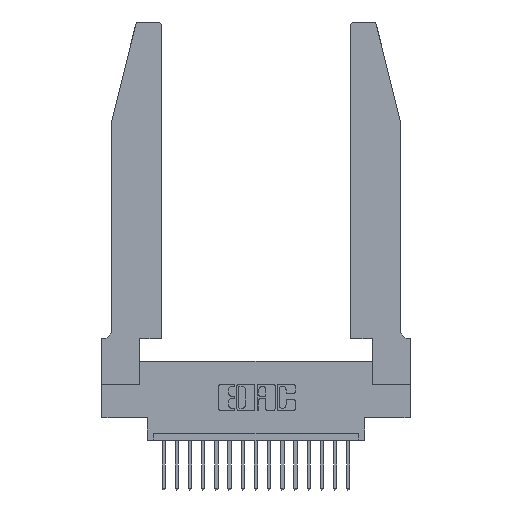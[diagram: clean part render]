
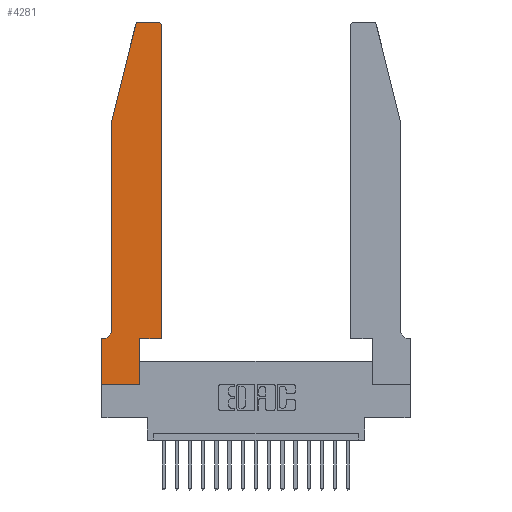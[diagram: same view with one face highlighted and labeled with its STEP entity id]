
A CAD part, top view. The second image highlights one B-rep face of the part: STEP entity #4281.
In plain terms, the highlighted planar face has unit normal (0, 0, 1).
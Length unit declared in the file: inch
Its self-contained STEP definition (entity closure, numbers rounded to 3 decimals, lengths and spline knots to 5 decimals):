
#148 = DIRECTION ( 'NONE',  ( 1., 0., 0. ) ) ;
#399 = CARTESIAN_POINT ( 'NONE',  ( 0., 0., 0.37 ) ) ;
#440 = ORIENTED_EDGE ( 'NONE', *, *, #5815, .T. ) ;
#626 = CARTESIAN_POINT ( 'NONE',  ( 0.4205, 2.75, 0.37 ) ) ;
#705 = CARTESIAN_POINT ( 'NONE',  ( 0.2865, 0., 0.37 ) ) ;
#860 = FACE_OUTER_BOUND ( 'NONE', #7319, .T. ) ;
#885 = VECTOR ( 'NONE', #10319, 39.37008 ) ;
#1140 = LINE ( 'NONE', #8821, #885 ) ;
#1640 = CARTESIAN_POINT ( 'NONE',  ( 0.2865, 0.35, 0.37 ) ) ;
#1805 = DIRECTION ( 'NONE',  ( 1., 0., 0. ) ) ;
#2067 = EDGE_CURVE ( 'NONE', #8173, #11769, #5464, .T. ) ;
#2202 = DIRECTION ( 'NONE',  ( 0., -1., 0. ) ) ;
#2368 = EDGE_CURVE ( 'NONE', #14955, #7671, #10485, .T. ) ;
#2386 = CARTESIAN_POINT ( 'NONE',  ( 0.0755, 0.42, 0.37 ) ) ;
#2513 = VECTOR ( 'NONE', #3049, 39.37008 ) ;
#2611 = CARTESIAN_POINT ( 'NONE',  ( 0., 0.35, 0.37 ) ) ;
#2957 = CARTESIAN_POINT ( 'NONE',  ( 0.4505, 0.35, 0.37 ) ) ;
#3036 = CARTESIAN_POINT ( 'NONE',  ( 0.4505, 2.72, 0.37 ) ) ;
#3049 = DIRECTION ( 'NONE',  ( 0., 1., 0. ) ) ;
#3166 = DIRECTION ( 'NONE',  ( -1., 0., 0. ) ) ;
#3198 = LINE ( 'NONE', #16047, #19476 ) ;
#3199 = VERTEX_POINT ( 'NONE', #17626 ) ;
#3205 = VECTOR ( 'NONE', #148, 39.37008 ) ;
#3424 = LINE ( 'NONE', #18947, #19233 ) ;
#3485 = LINE ( 'NONE', #18384, #2513 ) ;
#3638 = VERTEX_POINT ( 'NONE', #11807 ) ;
#3843 = VECTOR ( 'NONE', #16090, 39.37008 ) ;
#4262 = ORIENTED_EDGE ( 'NONE', *, *, #11011, .T. ) ;
#4281 = ADVANCED_FACE ( 'NONE', ( #860 ), #19414, .T. ) ;
#4558 = EDGE_CURVE ( 'NONE', #14735, #10683, #17620, .T. ) ;
#4709 = ORIENTED_EDGE ( 'NONE', *, *, #2368, .T. ) ;
#4916 = VECTOR ( 'NONE', #10738, 39.37008 ) ;
#5290 = CARTESIAN_POINT ( 'NONE',  ( 0.0755, 2., 0.37 ) ) ;
#5464 = LINE ( 'NONE', #12771, #7163 ) ;
#5568 = ORIENTED_EDGE ( 'NONE', *, *, #4558, .T. ) ;
#5815 = EDGE_CURVE ( 'NONE', #10683, #9415, #7547, .T. ) ;
#5868 = AXIS2_PLACEMENT_3D ( 'NONE', #6374, #7878, #3166 ) ;
#5882 = VECTOR ( 'NONE', #17864, 39.37008 ) ;
#6093 = CARTESIAN_POINT ( 'NONE',  ( 0.2865, 0.35, 0.37 ) ) ;
#6243 = DIRECTION ( 'NONE',  ( 1., 0., 0. ) ) ;
#6374 = CARTESIAN_POINT ( 'NONE',  ( 0.0055, 0.42, 0.37 ) ) ;
#6703 = EDGE_CURVE ( 'NONE', #12247, #3638, #7775, .T. ) ;
#7163 = VECTOR ( 'NONE', #2202, 39.37008 ) ;
#7184 = EDGE_CURVE ( 'NONE', #11769, #14735, #3424, .T. ) ;
#7208 = VERTEX_POINT ( 'NONE', #19222 ) ;
#7319 = EDGE_LOOP ( 'NONE', ( #17486, #10055, #15173, #14132, #19336, #10946, #9976, #7925, #5568, #440, #4262, #4709 ) ) ;
#7547 = LINE ( 'NONE', #13932, #3205 ) ;
#7671 = VERTEX_POINT ( 'NONE', #626 ) ;
#7775 = CIRCLE ( 'NONE', #5868, 0.07 ) ;
#7878 = DIRECTION ( 'NONE',  ( 0., 0., -1. ) ) ;
#7925 = ORIENTED_EDGE ( 'NONE', *, *, #7184, .T. ) ;
#8173 = VERTEX_POINT ( 'NONE', #11943 ) ;
#8486 = DIRECTION ( 'NONE',  ( 0., 0., 1. ) ) ;
#8821 = CARTESIAN_POINT ( 'NONE',  ( 0.2605, 2.75, 0.37 ) ) ;
#9415 = VERTEX_POINT ( 'NONE', #2957 ) ;
#9976 = ORIENTED_EDGE ( 'NONE', *, *, #2067, .T. ) ;
#10055 = ORIENTED_EDGE ( 'NONE', *, *, #19707, .T. ) ;
#10319 = DIRECTION ( 'NONE',  ( -1., 0., 0. ) ) ;
#10485 = CIRCLE ( 'NONE', #19024, 0.03 ) ;
#10683 = VERTEX_POINT ( 'NONE', #6093 ) ;
#10738 = DIRECTION ( 'NONE',  ( 0., 1., 0. ) ) ;
#10946 = ORIENTED_EDGE ( 'NONE', *, *, #12886, .T. ) ;
#11011 = EDGE_CURVE ( 'NONE', #9415, #14955, #3485, .T. ) ;
#11031 = DIRECTION ( 'NONE',  ( 1., 0., 0. ) ) ;
#11230 = LINE ( 'NONE', #5290, #3843 ) ;
#11444 = DIRECTION ( 'NONE',  ( 1., 0., 0. ) ) ;
#11611 = AXIS2_PLACEMENT_3D ( 'NONE', #13593, #12509, #1805 ) ;
#11769 = VERTEX_POINT ( 'NONE', #399 ) ;
#11807 = CARTESIAN_POINT ( 'NONE',  ( 0.0055, 0.35, 0.37 ) ) ;
#11943 = CARTESIAN_POINT ( 'NONE',  ( 0., 0.35, 0.37 ) ) ;
#12247 = VERTEX_POINT ( 'NONE', #2386 ) ;
#12509 = DIRECTION ( 'NONE',  ( 0., 0., 1. ) ) ;
#12771 = CARTESIAN_POINT ( 'NONE',  ( 0., 0., 0.37 ) ) ;
#12886 = EDGE_CURVE ( 'NONE', #3638, #8173, #3198, .T. ) ;
#13560 = DIRECTION ( 'NONE',  ( -1., 0., 0. ) ) ;
#13593 = CARTESIAN_POINT ( 'NONE',  ( 0.284, 2.72, 0.37 ) ) ;
#13790 = DIRECTION ( 'NONE',  ( 0., 0., 1. ) ) ;
#13932 = CARTESIAN_POINT ( 'NONE',  ( 0.4505, 0.35, 0.37 ) ) ;
#14132 = ORIENTED_EDGE ( 'NONE', *, *, #18335, .T. ) ;
#14729 = EDGE_CURVE ( 'NONE', #3199, #14953, #11230, .T. ) ;
#14735 = VERTEX_POINT ( 'NONE', #705 ) ;
#14953 = VERTEX_POINT ( 'NONE', #19846 ) ;
#14955 = VERTEX_POINT ( 'NONE', #3036 ) ;
#15143 = CARTESIAN_POINT ( 'NONE',  ( 0.4205, 2.72, 0.37 ) ) ;
#15173 = ORIENTED_EDGE ( 'NONE', *, *, #14729, .T. ) ;
#15403 = CIRCLE ( 'NONE', #11611, 0.03 ) ;
#16047 = CARTESIAN_POINT ( 'NONE',  ( 0.0755, 0.35, 0.37 ) ) ;
#16090 = DIRECTION ( 'NONE',  ( -0.239, -0.971, 0. ) ) ;
#16353 = CARTESIAN_POINT ( 'NONE',  ( 0.0755, 2., 0.37 ) ) ;
#16496 = EDGE_CURVE ( 'NONE', #7671, #7208, #1140, .T. ) ;
#17115 = LINE ( 'NONE', #16353, #5882 ) ;
#17486 = ORIENTED_EDGE ( 'NONE', *, *, #16496, .T. ) ;
#17620 = LINE ( 'NONE', #1640, #4916 ) ;
#17626 = CARTESIAN_POINT ( 'NONE',  ( 0.25487, 2.72718, 0.37 ) ) ;
#17864 = DIRECTION ( 'NONE',  ( 0., -1., 0. ) ) ;
#18335 = EDGE_CURVE ( 'NONE', #14953, #12247, #17115, .T. ) ;
#18384 = CARTESIAN_POINT ( 'NONE',  ( 0.4505, 0.35, 0.37 ) ) ;
#18947 = CARTESIAN_POINT ( 'NONE',  ( 0., 0., 0.37 ) ) ;
#19024 = AXIS2_PLACEMENT_3D ( 'NONE', #15143, #13790, #6243 ) ;
#19222 = CARTESIAN_POINT ( 'NONE',  ( 0.284, 2.75, 0.37 ) ) ;
#19233 = VECTOR ( 'NONE', #11444, 39.37008 ) ;
#19336 = ORIENTED_EDGE ( 'NONE', *, *, #6703, .T. ) ;
#19414 = PLANE ( 'NONE',  #19833 ) ;
#19476 = VECTOR ( 'NONE', #13560, 39.37008 ) ;
#19707 = EDGE_CURVE ( 'NONE', #7208, #3199, #15403, .T. ) ;
#19833 = AXIS2_PLACEMENT_3D ( 'NONE', #2611, #8486, #11031 ) ;
#19846 = CARTESIAN_POINT ( 'NONE',  ( 0.0755, 2., 0.37 ) ) ;
